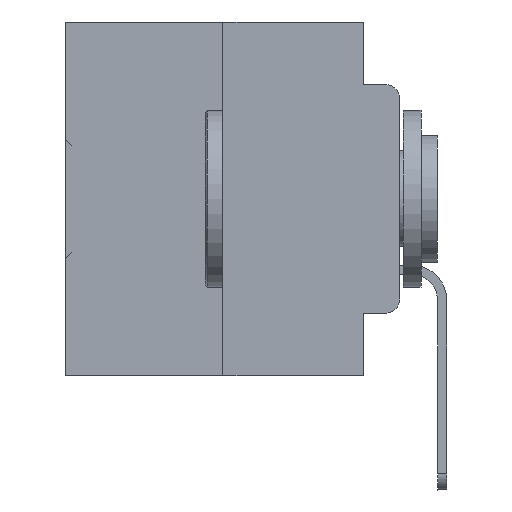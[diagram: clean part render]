
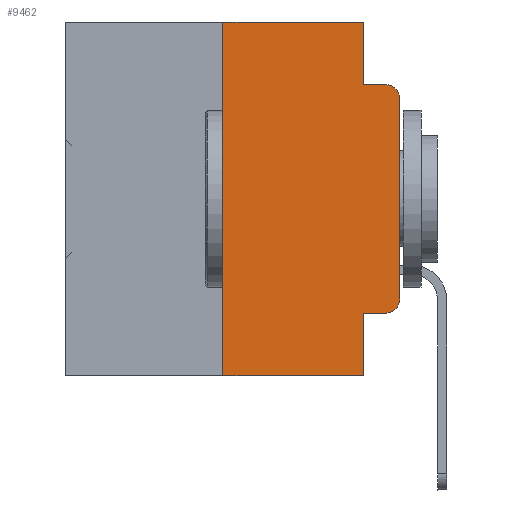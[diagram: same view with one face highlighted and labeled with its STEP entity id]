
A CAD part, left-side view. The second image highlights one B-rep face of the part: STEP entity #9462.
In plain terms, the highlighted planar face has unit normal (-1, 0, 0).
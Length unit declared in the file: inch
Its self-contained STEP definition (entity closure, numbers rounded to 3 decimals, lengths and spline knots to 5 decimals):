
#227 = VERTEX_POINT ( 'NONE', #27138 ) ;
#275 = EDGE_CURVE ( 'NONE', #24283, #15770, #8820, .T. ) ;
#393 = FACE_OUTER_BOUND ( 'NONE', #1915, .T. ) ;
#742 = AXIS2_PLACEMENT_3D ( 'NONE', #6870, #1032, #23590 ) ;
#811 = EDGE_CURVE ( 'NONE', #29928, #15601, #11615, .T. ) ;
#1032 = DIRECTION ( 'NONE',  ( -1., 0., 0. ) ) ;
#1559 = ORIENTED_EDGE ( 'NONE', *, *, #20839, .F. ) ;
#1827 = LINE ( 'NONE', #33060, #33874 ) ;
#1915 = EDGE_LOOP ( 'NONE', ( #11863, #33826, #1559, #25103, #11840, #29684, #8889, #6950, #19832, #11312 ) ) ;
#3449 = CARTESIAN_POINT ( 'NONE',  ( 0., 0., -0.1085 ) ) ;
#4250 = DIRECTION ( 'NONE',  ( -1., 0., 0. ) ) ;
#4293 = CARTESIAN_POINT ( 'NONE',  ( 0., 0.473, 0. ) ) ;
#4422 = VECTOR ( 'NONE', #9347, 39.37008 ) ;
#5834 = EDGE_CURVE ( 'NONE', #17534, #24283, #33791, .T. ) ;
#5844 = DIRECTION ( 'NONE',  ( 0., -1., 0. ) ) ;
#6403 = CARTESIAN_POINT ( 'NONE',  ( 0., 0.473, 0. ) ) ;
#6585 = DIRECTION ( 'NONE',  ( 1., 0., 0. ) ) ;
#6870 = CARTESIAN_POINT ( 'NONE',  ( 0., 0.02, -0.3915 ) ) ;
#6950 = ORIENTED_EDGE ( 'NONE', *, *, #811, .F. ) ;
#8820 = LINE ( 'NONE', #14465, #31455 ) ;
#8889 = ORIENTED_EDGE ( 'NONE', *, *, #29818, .T. ) ;
#9347 = DIRECTION ( 'NONE',  ( 0., 0., -1. ) ) ;
#9462 = ADVANCED_FACE ( 'NONE', ( #393 ), #11858, .F. ) ;
#11119 = EDGE_CURVE ( 'NONE', #227, #27525, #30013, .T. ) ;
#11312 = ORIENTED_EDGE ( 'NONE', *, *, #5834, .T. ) ;
#11615 = LINE ( 'NONE', #17797, #4422 ) ;
#11835 = VECTOR ( 'NONE', #23697, 39.37008 ) ;
#11840 = ORIENTED_EDGE ( 'NONE', *, *, #11119, .F. ) ;
#11858 = PLANE ( 'NONE',  #37195 ) ;
#11863 = ORIENTED_EDGE ( 'NONE', *, *, #275, .T. ) ;
#12229 = VERTEX_POINT ( 'NONE', #18845 ) ;
#12606 = LINE ( 'NONE', #23499, #11835 ) ;
#13985 = CARTESIAN_POINT ( 'NONE',  ( 0., 0.051, -0.5 ) ) ;
#14465 = CARTESIAN_POINT ( 'NONE',  ( 0., 0., 0. ) ) ;
#14511 = AXIS2_PLACEMENT_3D ( 'NONE', #29978, #4250, #27185 ) ;
#14916 = CARTESIAN_POINT ( 'NONE',  ( 0., 0.02, -0.4115 ) ) ;
#15601 = VERTEX_POINT ( 'NONE', #13985 ) ;
#15770 = VERTEX_POINT ( 'NONE', #3449 ) ;
#16367 = DIRECTION ( 'NONE',  ( 0., -1., 0. ) ) ;
#17507 = VECTOR ( 'NONE', #30307, 39.37008 ) ;
#17534 = VERTEX_POINT ( 'NONE', #14916 ) ;
#17797 = CARTESIAN_POINT ( 'NONE',  ( 0., 0.051, 0. ) ) ;
#18845 = CARTESIAN_POINT ( 'NONE',  ( 0., 0.051, -0.0885 ) ) ;
#18984 = CARTESIAN_POINT ( 'NONE',  ( 0., 0.051, -0.4115 ) ) ;
#19832 = ORIENTED_EDGE ( 'NONE', *, *, #37119, .T. ) ;
#19979 = DIRECTION ( 'NONE',  ( 0., -1., 0. ) ) ;
#20839 = EDGE_CURVE ( 'NONE', #12229, #30361, #28442, .T. ) ;
#21710 = VECTOR ( 'NONE', #19979, 39.37008 ) ;
#21844 = LINE ( 'NONE', #30482, #17507 ) ;
#21980 = CARTESIAN_POINT ( 'NONE',  ( 0., 0.051, -0.4115 ) ) ;
#22709 = CARTESIAN_POINT ( 'NONE',  ( 0., 0., -0.3915 ) ) ;
#23499 = CARTESIAN_POINT ( 'NONE',  ( 0., 0.473, -0.5 ) ) ;
#23590 = DIRECTION ( 'NONE',  ( 0., 0., -1. ) ) ;
#23697 = DIRECTION ( 'NONE',  ( 0., -1., 0. ) ) ;
#23873 = DIRECTION ( 'NONE',  ( 0., 0., -1. ) ) ;
#24283 = VERTEX_POINT ( 'NONE', #22709 ) ;
#24564 = CARTESIAN_POINT ( 'NONE',  ( 0., 0.25, -0.5 ) ) ;
#25103 = ORIENTED_EDGE ( 'NONE', *, *, #29439, .F. ) ;
#25908 = CIRCLE ( 'NONE', #14511, 0.02 ) ;
#26176 = CARTESIAN_POINT ( 'NONE',  ( 0., 0.051, -0.0885 ) ) ;
#27035 = EDGE_CURVE ( 'NONE', #30406, #227, #1827, .T. ) ;
#27138 = CARTESIAN_POINT ( 'NONE',  ( 0., 0.25, 0. ) ) ;
#27185 = DIRECTION ( 'NONE',  ( 0., 0., -1. ) ) ;
#27525 = VERTEX_POINT ( 'NONE', #30874 ) ;
#27783 = DIRECTION ( 'NONE',  ( 0., 0., 1. ) ) ;
#28442 = LINE ( 'NONE', #26176, #21710 ) ;
#29439 = EDGE_CURVE ( 'NONE', #27525, #12229, #21844, .T. ) ;
#29684 = ORIENTED_EDGE ( 'NONE', *, *, #27035, .F. ) ;
#29818 = EDGE_CURVE ( 'NONE', #30406, #15601, #12606, .T. ) ;
#29928 = VERTEX_POINT ( 'NONE', #21980 ) ;
#29978 = CARTESIAN_POINT ( 'NONE',  ( 0., 0.02, -0.1085 ) ) ;
#30013 = LINE ( 'NONE', #4293, #30729 ) ;
#30307 = DIRECTION ( 'NONE',  ( 0., 0., -1. ) ) ;
#30361 = VERTEX_POINT ( 'NONE', #30570 ) ;
#30406 = VERTEX_POINT ( 'NONE', #24564 ) ;
#30482 = CARTESIAN_POINT ( 'NONE',  ( 0., 0.051, 0. ) ) ;
#30570 = CARTESIAN_POINT ( 'NONE',  ( 0., 0.02, -0.0885 ) ) ;
#30620 = LINE ( 'NONE', #18984, #36155 ) ;
#30729 = VECTOR ( 'NONE', #5844, 39.37008 ) ;
#30874 = CARTESIAN_POINT ( 'NONE',  ( 0., 0.051, 0. ) ) ;
#31455 = VECTOR ( 'NONE', #35348, 39.37008 ) ;
#33060 = CARTESIAN_POINT ( 'NONE',  ( 0., 0.25, 0. ) ) ;
#33791 = CIRCLE ( 'NONE', #742, 0.02 ) ;
#33826 = ORIENTED_EDGE ( 'NONE', *, *, #35486, .T. ) ;
#33874 = VECTOR ( 'NONE', #27783, 39.37008 ) ;
#35348 = DIRECTION ( 'NONE',  ( 0., 0., 1. ) ) ;
#35486 = EDGE_CURVE ( 'NONE', #15770, #30361, #25908, .T. ) ;
#36155 = VECTOR ( 'NONE', #16367, 39.37008 ) ;
#37119 = EDGE_CURVE ( 'NONE', #29928, #17534, #30620, .T. ) ;
#37195 = AXIS2_PLACEMENT_3D ( 'NONE', #6403, #6585, #23873 ) ;
